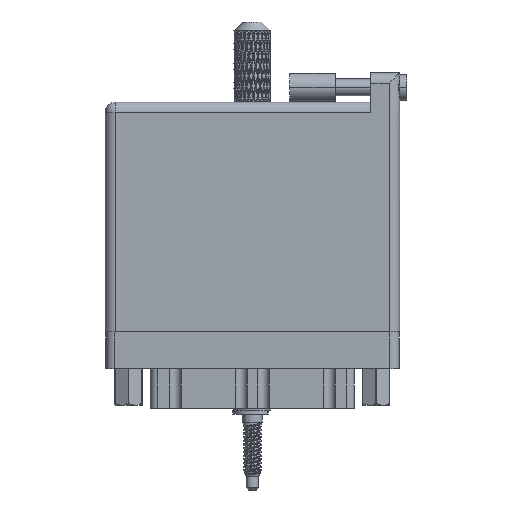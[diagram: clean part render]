
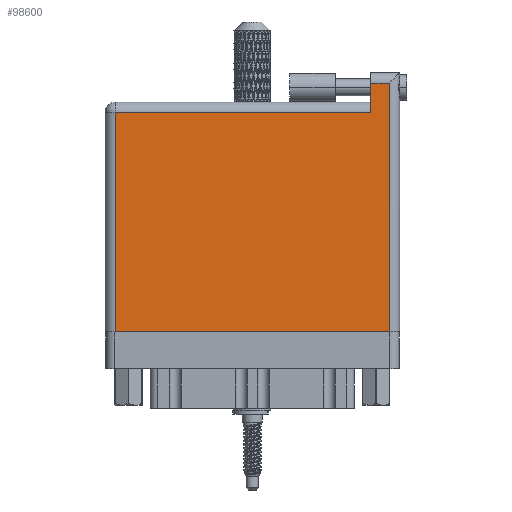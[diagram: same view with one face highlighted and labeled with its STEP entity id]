
A CAD part, front view. The second image highlights one B-rep face of the part: STEP entity #98600.
In plain terms, the highlighted face is planar.
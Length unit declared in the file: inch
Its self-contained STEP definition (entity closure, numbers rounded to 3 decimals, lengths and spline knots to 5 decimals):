
#917 = CARTESIAN_POINT ( 'NONE',  ( 0.07, 1.496, 0. ) ) ;
#3675 = DIRECTION ( 'NONE',  ( 0., 0., -1. ) ) ;
#5835 = ORIENTED_EDGE ( 'NONE', *, *, #47437, .T. ) ;
#7161 = CARTESIAN_POINT ( 'NONE',  ( 1.938, 0., 0. ) ) ;
#11926 = VECTOR ( 'NONE', #105900, 39.37008 ) ;
#14813 = VERTEX_POINT ( 'NONE', #917 ) ;
#17317 = VERTEX_POINT ( 'NONE', #42574 ) ;
#19914 = LINE ( 'NONE', #72003, #70574 ) ;
#20033 = LINE ( 'NONE', #80728, #11926 ) ;
#29509 = EDGE_LOOP ( 'NONE', ( #5835, #47514, #55923, #85578, #90071, #48690 ) ) ;
#30945 = EDGE_CURVE ( 'NONE', #111658, #14813, #20033, .T. ) ;
#32775 = VERTEX_POINT ( 'NONE', #97657 ) ;
#33495 = LINE ( 'NONE', #77016, #59208 ) ;
#33944 = VERTEX_POINT ( 'NONE', #7161 ) ;
#39495 = VECTOR ( 'NONE', #78910, 39.37008 ) ;
#41142 = DIRECTION ( 'NONE',  ( 0., -1., 0. ) ) ;
#41859 = EDGE_CURVE ( 'NONE', #75239, #111658, #104089, .T. ) ;
#42574 = CARTESIAN_POINT ( 'NONE',  ( 0.07, 0., 0. ) ) ;
#45529 = EDGE_CURVE ( 'NONE', #32775, #75239, #33495, .T. ) ;
#46228 = CARTESIAN_POINT ( 'NONE',  ( 0.07, 0., 0. ) ) ;
#47437 = EDGE_CURVE ( 'NONE', #17317, #33944, #78728, .T. ) ;
#47514 = ORIENTED_EDGE ( 'NONE', *, *, #110239, .T. ) ;
#48690 = ORIENTED_EDGE ( 'NONE', *, *, #112057, .T. ) ;
#52062 = VECTOR ( 'NONE', #52397, 39.37008 ) ;
#52390 = DIRECTION ( 'NONE',  ( -1., 0., 0. ) ) ;
#52397 = DIRECTION ( 'NONE',  ( 1., 0., 0. ) ) ;
#54804 = DIRECTION ( 'NONE',  ( 0., 1., 0. ) ) ;
#55923 = ORIENTED_EDGE ( 'NONE', *, *, #45529, .T. ) ;
#57815 = DIRECTION ( 'NONE',  ( -1., 0., 0. ) ) ;
#58848 = CARTESIAN_POINT ( 'NONE',  ( 1.811, 1.766, 0. ) ) ;
#59208 = VECTOR ( 'NONE', #52390, 39.37008 ) ;
#70574 = VECTOR ( 'NONE', #54804, 39.37008 ) ;
#71216 = CARTESIAN_POINT ( 'NONE',  ( 0., 1.566, 0. ) ) ;
#71775 = FACE_OUTER_BOUND ( 'NONE', #29509, .T. ) ;
#72003 = CARTESIAN_POINT ( 'NONE',  ( 1.938, 1.766, 0. ) ) ;
#75239 = VERTEX_POINT ( 'NONE', #83269 ) ;
#77016 = CARTESIAN_POINT ( 'NONE',  ( 0., 1.696, 0. ) ) ;
#77215 = AXIS2_PLACEMENT_3D ( 'NONE', #71216, #3675, #57815 ) ;
#78728 = LINE ( 'NONE', #89539, #52062 ) ;
#78910 = DIRECTION ( 'NONE',  ( 0., -1., 0. ) ) ;
#80728 = CARTESIAN_POINT ( 'NONE',  ( 0., 1.496, 0. ) ) ;
#80937 = PLANE ( 'NONE',  #77215 ) ;
#83269 = CARTESIAN_POINT ( 'NONE',  ( 1.811, 1.696, 0. ) ) ;
#85578 = ORIENTED_EDGE ( 'NONE', *, *, #41859, .T. ) ;
#89539 = CARTESIAN_POINT ( 'NONE',  ( 0., 0., 0. ) ) ;
#90071 = ORIENTED_EDGE ( 'NONE', *, *, #30945, .T. ) ;
#97657 = CARTESIAN_POINT ( 'NONE',  ( 1.938, 1.696, 0. ) ) ;
#98600 = ADVANCED_FACE ( 'NONE', ( #71775 ), #80937, .F. ) ;
#102880 = VECTOR ( 'NONE', #41142, 39.37008 ) ;
#104089 = LINE ( 'NONE', #58848, #102880 ) ;
#105900 = DIRECTION ( 'NONE',  ( -1., 0., 0. ) ) ;
#106875 = LINE ( 'NONE', #46228, #39495 ) ;
#110239 = EDGE_CURVE ( 'NONE', #33944, #32775, #19914, .T. ) ;
#111107 = CARTESIAN_POINT ( 'NONE',  ( 1.811, 1.496, 0. ) ) ;
#111658 = VERTEX_POINT ( 'NONE', #111107 ) ;
#112057 = EDGE_CURVE ( 'NONE', #14813, #17317, #106875, .T. ) ;
